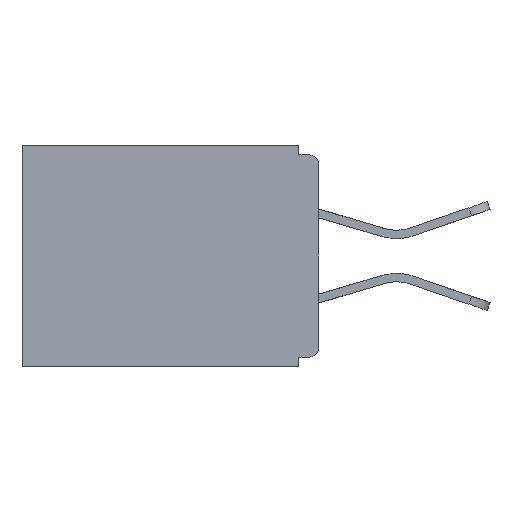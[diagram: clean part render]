
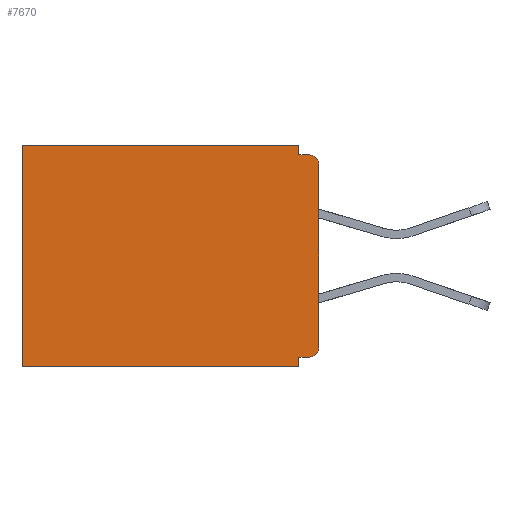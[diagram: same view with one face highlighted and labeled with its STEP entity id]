
A CAD part, left-side view. The second image highlights one B-rep face of the part: STEP entity #7670.
In plain terms, the highlighted planar face has unit normal (-1, 0, 0).
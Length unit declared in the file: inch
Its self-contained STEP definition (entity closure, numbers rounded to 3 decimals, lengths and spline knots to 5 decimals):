
#185 = LINE ( 'NONE', #10261, #14528 ) ;
#413 = CIRCLE ( 'NONE', #12511, 0.015 ) ;
#476 = DIRECTION ( 'NONE',  ( 0., 0., -1. ) ) ;
#481 = EDGE_CURVE ( 'NONE', #6197, #3444, #15025, .T. ) ;
#573 = CARTESIAN_POINT ( 'NONE',  ( 0.298, 0.015, -0.313 ) ) ;
#602 = AXIS2_PLACEMENT_3D ( 'NONE', #13070, #13220, #6096 ) ;
#634 = FACE_OUTER_BOUND ( 'NONE', #8760, .T. ) ;
#787 = CARTESIAN_POINT ( 'NONE',  ( 0.298, 0., -0.313 ) ) ;
#799 = CARTESIAN_POINT ( 'NONE',  ( 0.298, 0.031, -0.343 ) ) ;
#1263 = LINE ( 'NONE', #10344, #2550 ) ;
#1745 = CARTESIAN_POINT ( 'NONE',  ( 0.298, 0.46, 0. ) ) ;
#1938 = DIRECTION ( 'NONE',  ( -1., 0., 0. ) ) ;
#2204 = EDGE_CURVE ( 'NONE', #2738, #10719, #12392, .T. ) ;
#2504 = VERTEX_POINT ( 'NONE', #15972 ) ;
#2550 = VECTOR ( 'NONE', #15817, 39.37008 ) ;
#2632 = ORIENTED_EDGE ( 'NONE', *, *, #5810, .F. ) ;
#2675 = EDGE_CURVE ( 'NONE', #2979, #9608, #16219, .T. ) ;
#2738 = VERTEX_POINT ( 'NONE', #1745 ) ;
#2936 = EDGE_CURVE ( 'NONE', #2504, #14729, #185, .T. ) ;
#2979 = VERTEX_POINT ( 'NONE', #5018 ) ;
#3118 = ORIENTED_EDGE ( 'NONE', *, *, #8035, .F. ) ;
#3444 = VERTEX_POINT ( 'NONE', #16401 ) ;
#3616 = EDGE_CURVE ( 'NONE', #12917, #2738, #16661, .T. ) ;
#3675 = ORIENTED_EDGE ( 'NONE', *, *, #9686, .T. ) ;
#4181 = VERTEX_POINT ( 'NONE', #799 ) ;
#4235 = DIRECTION ( 'NONE',  ( 0., 0., -1. ) ) ;
#4559 = VECTOR ( 'NONE', #5431, 39.37008 ) ;
#5018 = CARTESIAN_POINT ( 'NONE',  ( 0.298, 0.015, -0.328 ) ) ;
#5032 = DIRECTION ( 'NONE',  ( 0., 1., 0. ) ) ;
#5054 = DIRECTION ( 'NONE',  ( 0., 0., -1. ) ) ;
#5420 = LINE ( 'NONE', #7045, #7752 ) ;
#5431 = DIRECTION ( 'NONE',  ( 0., 0., -1. ) ) ;
#5550 = CARTESIAN_POINT ( 'NONE',  ( 0.298, 0., -0.328 ) ) ;
#5556 = ORIENTED_EDGE ( 'NONE', *, *, #2204, .T. ) ;
#5661 = ORIENTED_EDGE ( 'NONE', *, *, #2675, .F. ) ;
#5810 = EDGE_CURVE ( 'NONE', #12917, #6197, #7390, .T. ) ;
#6096 = DIRECTION ( 'NONE',  ( 0., 0., -1. ) ) ;
#6161 = CARTESIAN_POINT ( 'NONE',  ( 0.298, 0., -0.015 ) ) ;
#6197 = VERTEX_POINT ( 'NONE', #15804 ) ;
#7045 = CARTESIAN_POINT ( 'NONE',  ( 0.298, 0.031, -0.343 ) ) ;
#7077 = EDGE_CURVE ( 'NONE', #9608, #4181, #5420, .T. ) ;
#7390 = LINE ( 'NONE', #12513, #8255 ) ;
#7605 = VECTOR ( 'NONE', #10081, 39.37008 ) ;
#7670 = ADVANCED_FACE ( 'NONE', ( #634 ), #14563, .F. ) ;
#7703 = VECTOR ( 'NONE', #16660, 39.37008 ) ;
#7752 = VECTOR ( 'NONE', #4235, 39.37008 ) ;
#8035 = EDGE_CURVE ( 'NONE', #4181, #10719, #1263, .T. ) ;
#8111 = ORIENTED_EDGE ( 'NONE', *, *, #7077, .F. ) ;
#8255 = VECTOR ( 'NONE', #13876, 39.37008 ) ;
#8333 = ORIENTED_EDGE ( 'NONE', *, *, #2936, .F. ) ;
#8760 = EDGE_LOOP ( 'NONE', ( #3675, #13445, #2632, #10748, #5556, #3118, #8111, #5661, #13015, #8333 ) ) ;
#9112 = CIRCLE ( 'NONE', #9226, 0.015 ) ;
#9226 = AXIS2_PLACEMENT_3D ( 'NONE', #573, #1938, #5054 ) ;
#9263 = VECTOR ( 'NONE', #5032, 39.37008 ) ;
#9608 = VERTEX_POINT ( 'NONE', #15434 ) ;
#9686 = EDGE_CURVE ( 'NONE', #2504, #3444, #413, .T. ) ;
#9946 = CARTESIAN_POINT ( 'NONE',  ( 0.298, 0.031, 0. ) ) ;
#10081 = DIRECTION ( 'NONE',  ( 0., -1., 0. ) ) ;
#10261 = CARTESIAN_POINT ( 'NONE',  ( 0.298, 0., 0. ) ) ;
#10331 = CARTESIAN_POINT ( 'NONE',  ( 0.298, 0., 0. ) ) ;
#10344 = CARTESIAN_POINT ( 'NONE',  ( 0.298, 0., -0.343 ) ) ;
#10719 = VERTEX_POINT ( 'NONE', #14829 ) ;
#10748 = ORIENTED_EDGE ( 'NONE', *, *, #3616, .T. ) ;
#11485 = DIRECTION ( 'NONE',  ( -1., 0., 0. ) ) ;
#12325 = CARTESIAN_POINT ( 'NONE',  ( 0.298, 0.46, 0. ) ) ;
#12392 = LINE ( 'NONE', #12325, #4559 ) ;
#12511 = AXIS2_PLACEMENT_3D ( 'NONE', #17059, #11485, #16992 ) ;
#12513 = CARTESIAN_POINT ( 'NONE',  ( 0.298, 0.031, -0.343 ) ) ;
#12917 = VERTEX_POINT ( 'NONE', #9946 ) ;
#13015 = ORIENTED_EDGE ( 'NONE', *, *, #15934, .T. ) ;
#13070 = CARTESIAN_POINT ( 'NONE',  ( 0.298, 0., 0. ) ) ;
#13220 = DIRECTION ( 'NONE',  ( 1., 0., 0. ) ) ;
#13445 = ORIENTED_EDGE ( 'NONE', *, *, #481, .F. ) ;
#13876 = DIRECTION ( 'NONE',  ( 0., 0., -1. ) ) ;
#14528 = VECTOR ( 'NONE', #476, 39.37008 ) ;
#14563 = PLANE ( 'NONE',  #602 ) ;
#14729 = VERTEX_POINT ( 'NONE', #787 ) ;
#14829 = CARTESIAN_POINT ( 'NONE',  ( 0.298, 0.46, -0.343 ) ) ;
#15025 = LINE ( 'NONE', #6161, #7605 ) ;
#15434 = CARTESIAN_POINT ( 'NONE',  ( 0.298, 0.031, -0.328 ) ) ;
#15804 = CARTESIAN_POINT ( 'NONE',  ( 0.298, 0.031, -0.015 ) ) ;
#15817 = DIRECTION ( 'NONE',  ( 0., 1., 0. ) ) ;
#15934 = EDGE_CURVE ( 'NONE', #2979, #14729, #9112, .T. ) ;
#15972 = CARTESIAN_POINT ( 'NONE',  ( 0.298, 0., -0.03 ) ) ;
#16219 = LINE ( 'NONE', #5550, #7703 ) ;
#16401 = CARTESIAN_POINT ( 'NONE',  ( 0.298, 0.015, -0.015 ) ) ;
#16660 = DIRECTION ( 'NONE',  ( 0., 1., 0. ) ) ;
#16661 = LINE ( 'NONE', #10331, #9263 ) ;
#16992 = DIRECTION ( 'NONE',  ( 0., 0., -1. ) ) ;
#17059 = CARTESIAN_POINT ( 'NONE',  ( 0.298, 0.015, -0.03 ) ) ;
